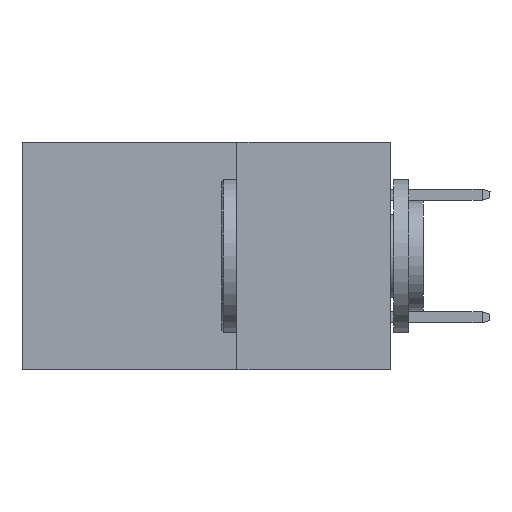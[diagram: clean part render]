
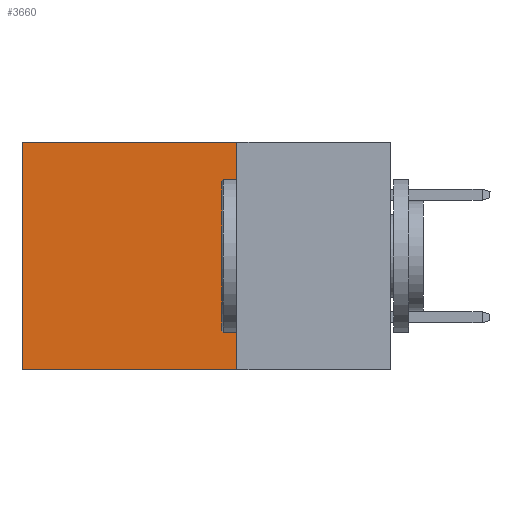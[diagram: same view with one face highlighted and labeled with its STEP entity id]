
A CAD part, left-side view. The second image highlights one B-rep face of the part: STEP entity #3660.
In plain terms, the highlighted planar face has unit normal (-1, 0, 0).
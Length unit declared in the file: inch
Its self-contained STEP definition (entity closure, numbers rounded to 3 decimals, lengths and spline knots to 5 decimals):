
#125 = DIRECTION ( 'NONE',  ( 0., 1., 0. ) ) ;
#275 = AXIS2_PLACEMENT_3D ( 'NONE', #3576, #8112, #4380 ) ;
#482 = LINE ( 'NONE', #2533, #5159 ) ;
#700 = VECTOR ( 'NONE', #9509, 39.37008 ) ;
#810 = VECTOR ( 'NONE', #5322, 39.37008 ) ;
#995 = VERTEX_POINT ( 'NONE', #7131 ) ;
#1826 = VERTEX_POINT ( 'NONE', #3665 ) ;
#2007 = VERTEX_POINT ( 'NONE', #3594 ) ;
#2287 = EDGE_CURVE ( 'NONE', #995, #1826, #2791, .T. ) ;
#2317 = LINE ( 'NONE', #6265, #700 ) ;
#2533 = CARTESIAN_POINT ( 'NONE',  ( 0.2875, 0.25, 0. ) ) ;
#2642 = FACE_OUTER_BOUND ( 'NONE', #6380, .T. ) ;
#2791 = LINE ( 'NONE', #3828, #810 ) ;
#2924 = EDGE_CURVE ( 'NONE', #2007, #1826, #2317, .T. ) ;
#3576 = CARTESIAN_POINT ( 'NONE',  ( 0.2875, 0.25, 0. ) ) ;
#3594 = CARTESIAN_POINT ( 'NONE',  ( 0.2875, 0.6, 0. ) ) ;
#3660 = ADVANCED_FACE ( 'NONE', ( #2642 ), #5043, .F. ) ;
#3665 = CARTESIAN_POINT ( 'NONE',  ( 0.2875, 0.6, -0.37 ) ) ;
#3828 = CARTESIAN_POINT ( 'NONE',  ( 0.2875, 0.25, -0.37 ) ) ;
#3884 = ORIENTED_EDGE ( 'NONE', *, *, #8600, .F. ) ;
#3918 = CARTESIAN_POINT ( 'NONE',  ( 0.2875, 0.25, 0. ) ) ;
#4040 = ORIENTED_EDGE ( 'NONE', *, *, #2287, .F. ) ;
#4380 = DIRECTION ( 'NONE',  ( 0., 0., -1. ) ) ;
#4481 = VECTOR ( 'NONE', #125, 39.37008 ) ;
#5043 = PLANE ( 'NONE',  #275 ) ;
#5159 = VECTOR ( 'NONE', #9260, 39.37008 ) ;
#5322 = DIRECTION ( 'NONE',  ( 0., 1., 0. ) ) ;
#6265 = CARTESIAN_POINT ( 'NONE',  ( 0.2875, 0.6, 0. ) ) ;
#6360 = ORIENTED_EDGE ( 'NONE', *, *, #7412, .T. ) ;
#6380 = EDGE_LOOP ( 'NONE', ( #9122, #4040, #3884, #6360 ) ) ;
#7131 = CARTESIAN_POINT ( 'NONE',  ( 0.2875, 0.25, -0.37 ) ) ;
#7412 = EDGE_CURVE ( 'NONE', #7613, #2007, #8894, .T. ) ;
#7613 = VERTEX_POINT ( 'NONE', #7925 ) ;
#7925 = CARTESIAN_POINT ( 'NONE',  ( 0.2875, 0.25, 0. ) ) ;
#8112 = DIRECTION ( 'NONE',  ( 1., 0., 0. ) ) ;
#8600 = EDGE_CURVE ( 'NONE', #7613, #995, #482, .T. ) ;
#8894 = LINE ( 'NONE', #3918, #4481 ) ;
#9122 = ORIENTED_EDGE ( 'NONE', *, *, #2924, .T. ) ;
#9260 = DIRECTION ( 'NONE',  ( 0., 0., -1. ) ) ;
#9509 = DIRECTION ( 'NONE',  ( 0., 0., -1. ) ) ;
